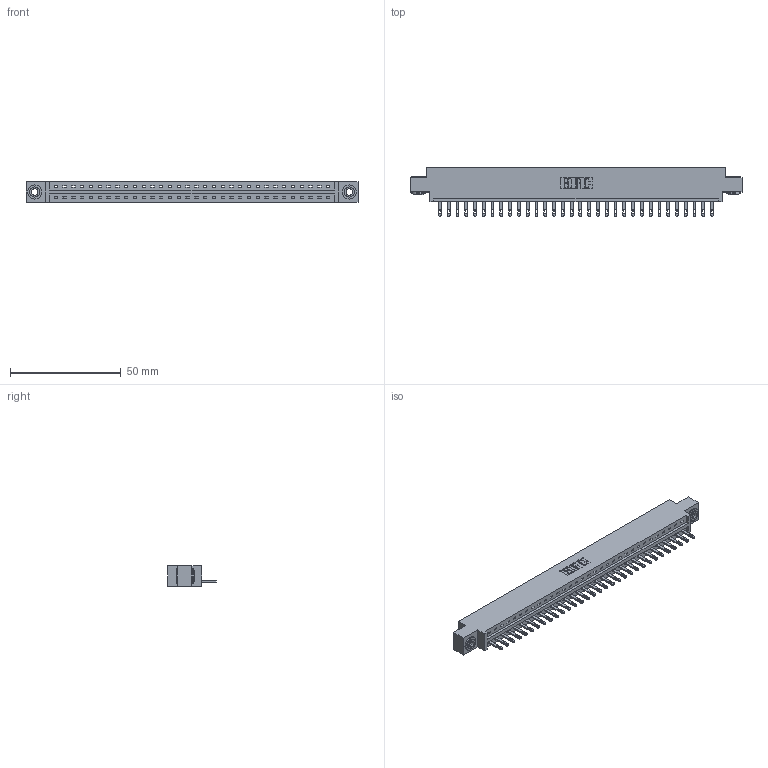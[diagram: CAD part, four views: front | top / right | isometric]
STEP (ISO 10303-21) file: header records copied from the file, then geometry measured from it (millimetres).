
FILE_DESCRIPTION (( 'STEP AP203' ), '1' );
FILE_NAME ('337-032-500-603.STEP', '2018-08-07T04:21:53', ( '' ), ( '' ), 'SwSTEP 2.0', 'SolidWorks 2016', '' );
FILE_SCHEMA (( 'CONFIG_CONTROL_DESIGN' ));
Length unit declared in the file: inch
Products named in the file (4): 345-292-001_345-293-100; 337 Part_0.170 Offset - 0.156 Dia-TH; 345-250-002_345-250-002-102; 337-032-500-603
Assembly tree (35 placements, depth 2):
  337-032-500-603
    337 Part_0.170 Offset - 0.156 Dia-TH
    345-292-001_345-293-100  x32
    345-250-002_345-250-002-102  x2
Bounding box: 149.81 x 21.85 x 9.4 mm (x, y, z)
Volume: 15366.7 mm3; surface area: 16227.6 mm2
Topology: 35 solids, 35 shells, 2012 faces, 6159 edges, 4102 vertices
Faces by surface type: plane 1364, cylinder 640, cone 8
Entity records: 25792 total; most frequent: CARTESIAN_POINT 4469, ORIENTED_EDGE 4430, DIRECTION 3817, EDGE_CURVE 2215, LINE 2059, VECTOR 2059, VERTEX_POINT 1474, AXIS2_PLACEMENT_3D 879
